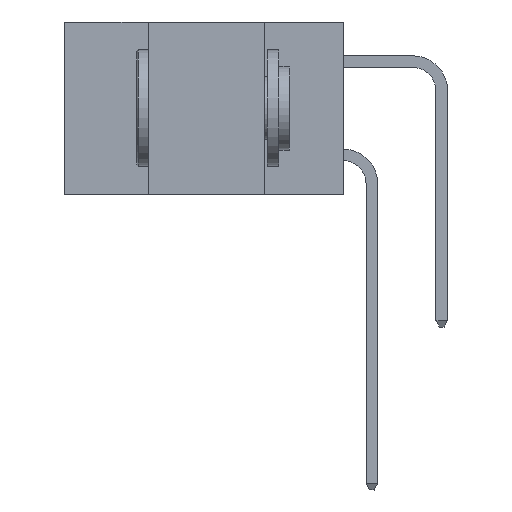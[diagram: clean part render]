
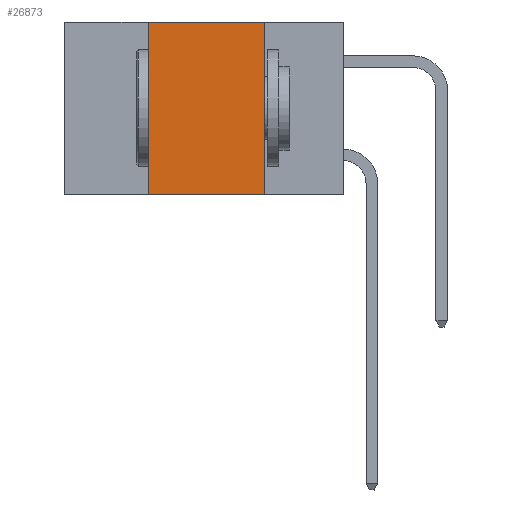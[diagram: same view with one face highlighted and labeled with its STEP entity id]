
A CAD part, left-side view. The second image highlights one B-rep face of the part: STEP entity #26873.
In plain terms, the highlighted planar face has unit normal (-1, 0, 0).
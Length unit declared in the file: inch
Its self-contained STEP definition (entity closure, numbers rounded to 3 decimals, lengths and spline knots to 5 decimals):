
#1719 = CARTESIAN_POINT ( 'NONE',  ( 0., 0.42, 0. ) ) ;
#4676 = EDGE_CURVE ( 'NONE', #21277, #6248, #8798, .T. ) ;
#4867 = VECTOR ( 'NONE', #22245, 39.37008 ) ;
#5323 = CARTESIAN_POINT ( 'NONE',  ( 0., 0.17, 0. ) ) ;
#5737 = EDGE_CURVE ( 'NONE', #14530, #21277, #22310, .T. ) ;
#6248 = VERTEX_POINT ( 'NONE', #16972 ) ;
#7604 = DIRECTION ( 'NONE',  ( 0., 0., -1. ) ) ;
#7628 = DIRECTION ( 'NONE',  ( 0., -1., 0. ) ) ;
#8522 = CARTESIAN_POINT ( 'NONE',  ( 0., 0.6, 0. ) ) ;
#8798 = LINE ( 'NONE', #8522, #14158 ) ;
#10322 = LINE ( 'NONE', #14407, #17143 ) ;
#10475 = DIRECTION ( 'NONE',  ( 1., 0., 0. ) ) ;
#11254 = EDGE_CURVE ( 'NONE', #6248, #13121, #20299, .T. ) ;
#13121 = VERTEX_POINT ( 'NONE', #18357 ) ;
#14158 = VECTOR ( 'NONE', #26983, 39.37008 ) ;
#14407 = CARTESIAN_POINT ( 'NONE',  ( 0., 0.6, -0.37 ) ) ;
#14530 = VERTEX_POINT ( 'NONE', #20537 ) ;
#16972 = CARTESIAN_POINT ( 'NONE',  ( 0., 0.17, 0. ) ) ;
#17143 = VECTOR ( 'NONE', #7628, 39.37008 ) ;
#18312 = FACE_OUTER_BOUND ( 'NONE', #19835, .T. ) ;
#18357 = CARTESIAN_POINT ( 'NONE',  ( 0., 0.17, -0.37 ) ) ;
#19547 = PLANE ( 'NONE',  #20838 ) ;
#19835 = EDGE_LOOP ( 'NONE', ( #27392, #21096, #22501, #25339 ) ) ;
#20299 = LINE ( 'NONE', #5323, #25585 ) ;
#20537 = CARTESIAN_POINT ( 'NONE',  ( 0., 0.42, -0.37 ) ) ;
#20838 = AXIS2_PLACEMENT_3D ( 'NONE', #24125, #10475, #26359 ) ;
#20981 = EDGE_CURVE ( 'NONE', #14530, #13121, #10322, .T. ) ;
#21096 = ORIENTED_EDGE ( 'NONE', *, *, #4676, .F. ) ;
#21277 = VERTEX_POINT ( 'NONE', #1719 ) ;
#22245 = DIRECTION ( 'NONE',  ( 0., 0., 1. ) ) ;
#22310 = LINE ( 'NONE', #24388, #4867 ) ;
#22501 = ORIENTED_EDGE ( 'NONE', *, *, #5737, .F. ) ;
#24125 = CARTESIAN_POINT ( 'NONE',  ( 0., 0.6, 0. ) ) ;
#24388 = CARTESIAN_POINT ( 'NONE',  ( 0., 0.42, 0. ) ) ;
#25339 = ORIENTED_EDGE ( 'NONE', *, *, #20981, .T. ) ;
#25585 = VECTOR ( 'NONE', #7604, 39.37008 ) ;
#26359 = DIRECTION ( 'NONE',  ( 0., 0., -1. ) ) ;
#26873 = ADVANCED_FACE ( 'NONE', ( #18312 ), #19547, .F. ) ;
#26983 = DIRECTION ( 'NONE',  ( 0., -1., 0. ) ) ;
#27392 = ORIENTED_EDGE ( 'NONE', *, *, #11254, .F. ) ;
